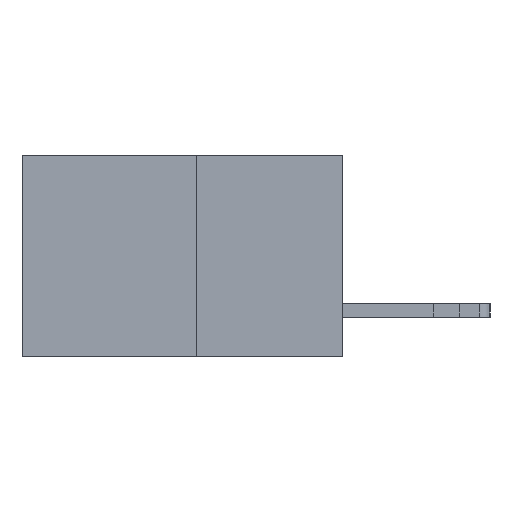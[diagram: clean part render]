
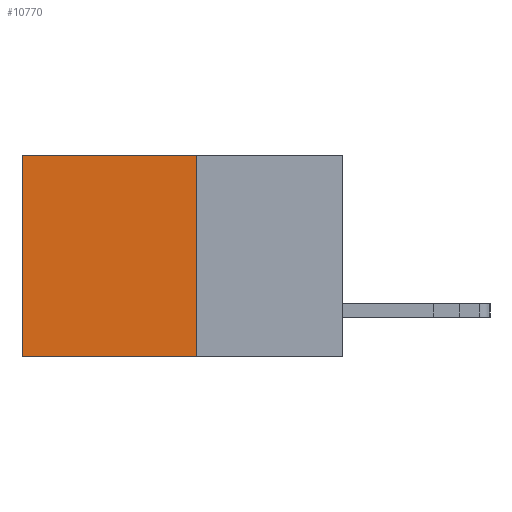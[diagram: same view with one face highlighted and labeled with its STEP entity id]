
A CAD part, left-side view. The second image highlights one B-rep face of the part: STEP entity #10770.
In plain terms, the highlighted planar face has unit normal (-1, 0, 0).
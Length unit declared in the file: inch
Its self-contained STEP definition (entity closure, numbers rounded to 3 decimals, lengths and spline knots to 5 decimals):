
#517 = CARTESIAN_POINT ( 'NONE',  ( 0.277, 0.27, -0.37 ) ) ;
#1503 = EDGE_CURVE ( 'NONE', #9123, #9668, #7044, .T. ) ;
#1607 = CARTESIAN_POINT ( 'NONE',  ( 0.277, 0.59, -0.37 ) ) ;
#1893 = DIRECTION ( 'NONE',  ( 1., 0., 0. ) ) ;
#2191 = DIRECTION ( 'NONE',  ( 0., 0., -1. ) ) ;
#2503 = CARTESIAN_POINT ( 'NONE',  ( 0.277, 0.59, 0. ) ) ;
#2746 = ORIENTED_EDGE ( 'NONE', *, *, #1503, .T. ) ;
#2877 = VECTOR ( 'NONE', #6560, 39.37008 ) ;
#3177 = VERTEX_POINT ( 'NONE', #4521 ) ;
#3726 = CARTESIAN_POINT ( 'NONE',  ( 0.277, 0.59, -0.37 ) ) ;
#4521 = CARTESIAN_POINT ( 'NONE',  ( 0.277, 0.27, 0. ) ) ;
#5141 = CARTESIAN_POINT ( 'NONE',  ( 0.277, 0.27, -0.37 ) ) ;
#6027 = FACE_OUTER_BOUND ( 'NONE', #13535, .T. ) ;
#6259 = PLANE ( 'NONE',  #14057 ) ;
#6560 = DIRECTION ( 'NONE',  ( 0., 0., -1. ) ) ;
#7044 = LINE ( 'NONE', #1607, #8332 ) ;
#8260 = VECTOR ( 'NONE', #10778, 39.37008 ) ;
#8332 = VECTOR ( 'NONE', #2191, 39.37008 ) ;
#8857 = CARTESIAN_POINT ( 'NONE',  ( 0.277, 0.27, 0. ) ) ;
#9123 = VERTEX_POINT ( 'NONE', #2503 ) ;
#9625 = EDGE_CURVE ( 'NONE', #3177, #12733, #10789, .T. ) ;
#9668 = VERTEX_POINT ( 'NONE', #3726 ) ;
#10385 = CARTESIAN_POINT ( 'NONE',  ( 0.277, 0.27, -0.37 ) ) ;
#10770 = ADVANCED_FACE ( 'NONE', ( #6027 ), #6259, .F. ) ;
#10778 = DIRECTION ( 'NONE',  ( 0., 1., 0. ) ) ;
#10789 = LINE ( 'NONE', #5141, #2877 ) ;
#11530 = ORIENTED_EDGE ( 'NONE', *, *, #15963, .T. ) ;
#11745 = DIRECTION ( 'NONE',  ( 0., 0., -1. ) ) ;
#12733 = VERTEX_POINT ( 'NONE', #517 ) ;
#12932 = DIRECTION ( 'NONE',  ( 0., 1., 0. ) ) ;
#13535 = EDGE_LOOP ( 'NONE', ( #2746, #17202, #16659, #11530 ) ) ;
#14057 = AXIS2_PLACEMENT_3D ( 'NONE', #10385, #1893, #11745 ) ;
#14883 = VECTOR ( 'NONE', #12932, 39.37008 ) ;
#15253 = LINE ( 'NONE', #17436, #8260 ) ;
#15298 = LINE ( 'NONE', #8857, #14883 ) ;
#15963 = EDGE_CURVE ( 'NONE', #3177, #9123, #15298, .T. ) ;
#16659 = ORIENTED_EDGE ( 'NONE', *, *, #9625, .F. ) ;
#17176 = EDGE_CURVE ( 'NONE', #12733, #9668, #15253, .T. ) ;
#17202 = ORIENTED_EDGE ( 'NONE', *, *, #17176, .F. ) ;
#17436 = CARTESIAN_POINT ( 'NONE',  ( 0.277, 0.27, -0.37 ) ) ;
